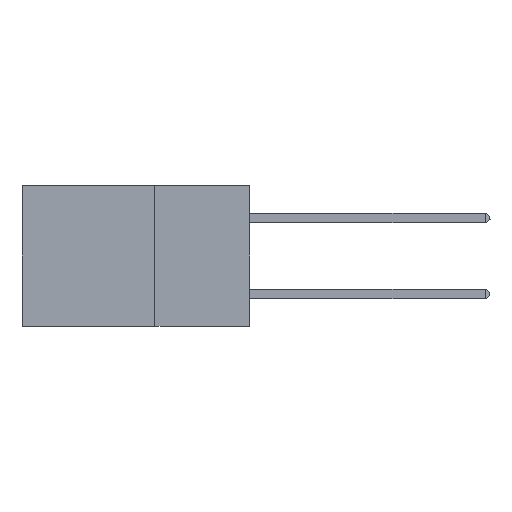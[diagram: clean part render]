
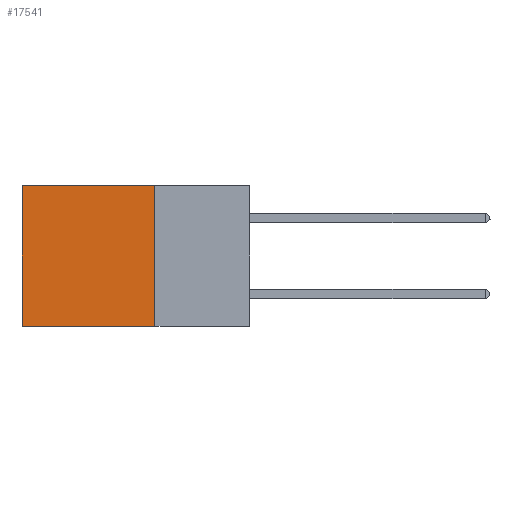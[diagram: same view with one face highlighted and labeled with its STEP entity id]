
A CAD part, left-side view. The second image highlights one B-rep face of the part: STEP entity #17541.
In plain terms, the highlighted planar face has unit normal (-1, 0, 0).
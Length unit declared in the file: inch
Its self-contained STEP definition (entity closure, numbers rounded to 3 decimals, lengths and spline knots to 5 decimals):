
#105 = VECTOR ( 'NONE', #16586, 39.37008 ) ;
#307 = CARTESIAN_POINT ( 'NONE',  ( 0.2875, 0.25, 0. ) ) ;
#829 = VERTEX_POINT ( 'NONE', #16365 ) ;
#1166 = EDGE_CURVE ( 'NONE', #8012, #829, #4415, .T. ) ;
#1204 = CARTESIAN_POINT ( 'NONE',  ( 0.2875, 0.25, 0. ) ) ;
#1639 = FACE_OUTER_BOUND ( 'NONE', #2057, .T. ) ;
#2057 = EDGE_LOOP ( 'NONE', ( #6791, #3984, #14635, #7035 ) ) ;
#2224 = CARTESIAN_POINT ( 'NONE',  ( 0.2875, 0.25, -0.37 ) ) ;
#2901 = DIRECTION ( 'NONE',  ( 0., 1., 0. ) ) ;
#3457 = DIRECTION ( 'NONE',  ( 0., 0., -1. ) ) ;
#3809 = LINE ( 'NONE', #10511, #13344 ) ;
#3984 = ORIENTED_EDGE ( 'NONE', *, *, #18368, .F. ) ;
#4415 = LINE ( 'NONE', #1204, #4504 ) ;
#4504 = VECTOR ( 'NONE', #2901, 39.37008 ) ;
#4754 = PLANE ( 'NONE',  #7557 ) ;
#4861 = DIRECTION ( 'NONE',  ( 1., 0., 0. ) ) ;
#5113 = VERTEX_POINT ( 'NONE', #12713 ) ;
#5547 = DIRECTION ( 'NONE',  ( 0., 1., 0. ) ) ;
#6673 = CARTESIAN_POINT ( 'NONE',  ( 0.2875, 0.25, 0. ) ) ;
#6791 = ORIENTED_EDGE ( 'NONE', *, *, #21055, .T. ) ;
#7035 = ORIENTED_EDGE ( 'NONE', *, *, #1166, .T. ) ;
#7557 = AXIS2_PLACEMENT_3D ( 'NONE', #6673, #4861, #3457 ) ;
#7573 = VECTOR ( 'NONE', #5547, 39.37008 ) ;
#8012 = VERTEX_POINT ( 'NONE', #307 ) ;
#8169 = CARTESIAN_POINT ( 'NONE',  ( 0.2875, 0.6, 0. ) ) ;
#10511 = CARTESIAN_POINT ( 'NONE',  ( 0.2875, 0.25, 0. ) ) ;
#11080 = CARTESIAN_POINT ( 'NONE',  ( 0.2875, 0.25, -0.37 ) ) ;
#12713 = CARTESIAN_POINT ( 'NONE',  ( 0.2875, 0.6, -0.37 ) ) ;
#13148 = VERTEX_POINT ( 'NONE', #11080 ) ;
#13344 = VECTOR ( 'NONE', #15532, 39.37008 ) ;
#14635 = ORIENTED_EDGE ( 'NONE', *, *, #19566, .F. ) ;
#15532 = DIRECTION ( 'NONE',  ( 0., 0., -1. ) ) ;
#16169 = LINE ( 'NONE', #8169, #105 ) ;
#16365 = CARTESIAN_POINT ( 'NONE',  ( 0.2875, 0.6, 0. ) ) ;
#16586 = DIRECTION ( 'NONE',  ( 0., 0., -1. ) ) ;
#17541 = ADVANCED_FACE ( 'NONE', ( #1639 ), #4754, .F. ) ;
#18368 = EDGE_CURVE ( 'NONE', #13148, #5113, #20003, .T. ) ;
#19566 = EDGE_CURVE ( 'NONE', #8012, #13148, #3809, .T. ) ;
#20003 = LINE ( 'NONE', #2224, #7573 ) ;
#21055 = EDGE_CURVE ( 'NONE', #829, #5113, #16169, .T. ) ;
